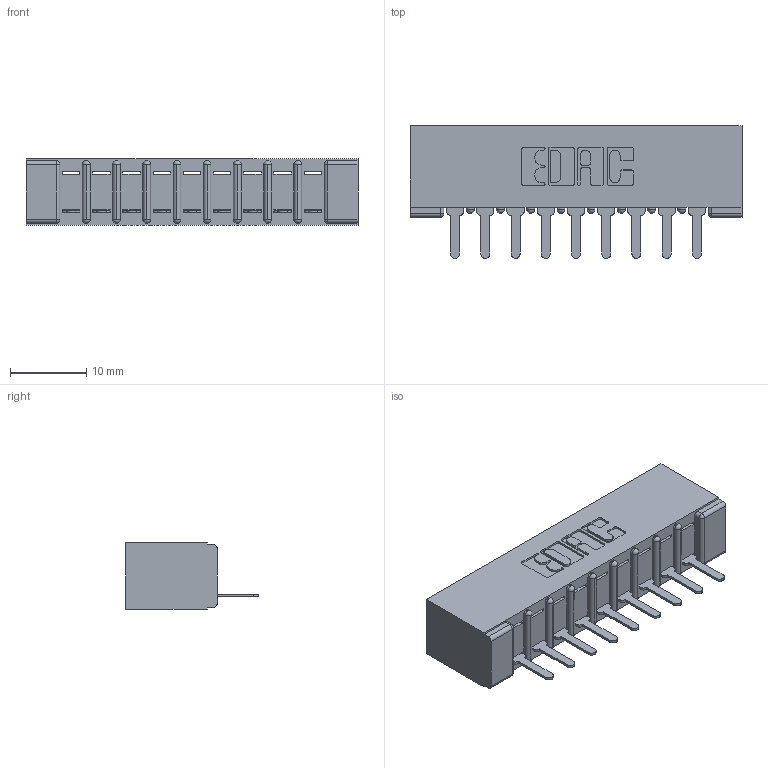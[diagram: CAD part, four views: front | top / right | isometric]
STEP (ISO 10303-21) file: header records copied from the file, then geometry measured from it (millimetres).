
FILE_DESCRIPTION (( 'STEP AP203' ), '1' );
FILE_NAME ('307-009-425-101.STEP', '2020-09-25T04:48:59', ( '' ), ( '' ), 'SwSTEP 2.0', 'SolidWorks 2020', '' );
FILE_SCHEMA (( 'CONFIG_CONTROL_DESIGN' ));
Length unit declared in the file: inch
Products named in the file (3): 307-290-001_525; 307 Part_No Mounting Lugs; 307-009-425-101
Assembly tree (10 placements, depth 2):
  307-009-425-101
    307 Part_No Mounting Lugs
    307-290-001_525  x9
Bounding box: 43.54 x 17.42 x 8.71 mm (x, y, z)
Volume: 2972.7 mm3; surface area: 4382.6 mm2
Topology: 10 solids, 10 shells, 624 faces, 1757 edges, 1130 vertices
Faces by surface type: plane 399, cylinder 205, sphere 20
Entity records: 11474 total; most frequent: CARTESIAN_POINT 1920, ORIENTED_EDGE 1906, DIRECTION 1885, EDGE_CURVE 953, VECTOR 719, LINE 719, VERTEX_POINT 618, AXIS2_PLACEMENT_3D 583
